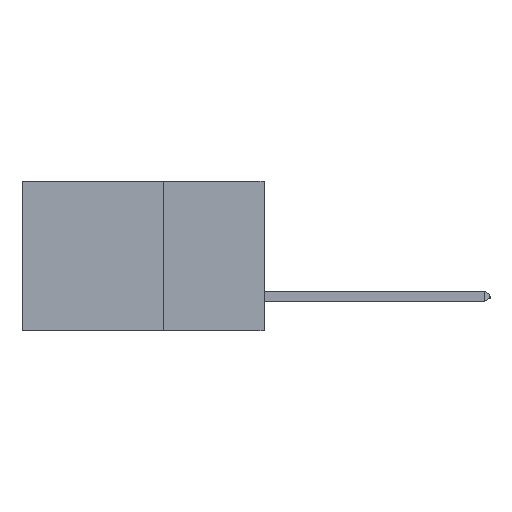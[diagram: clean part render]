
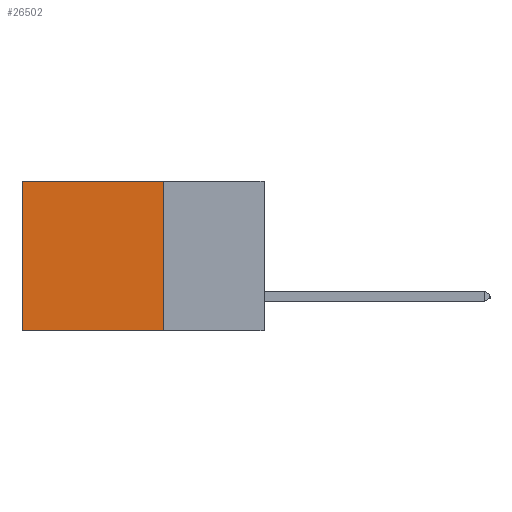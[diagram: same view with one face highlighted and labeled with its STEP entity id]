
A CAD part, left-side view. The second image highlights one B-rep face of the part: STEP entity #26502.
In plain terms, the highlighted planar face has unit normal (-1, 0, 0).
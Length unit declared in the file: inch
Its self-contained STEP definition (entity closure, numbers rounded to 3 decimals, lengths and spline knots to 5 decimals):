
#338 = CARTESIAN_POINT ( 'NONE',  ( 0.298, 0.25, -0.37 ) ) ;
#1048 = CARTESIAN_POINT ( 'NONE',  ( 0.298, 0.6, -0.37 ) ) ;
#1110 = CARTESIAN_POINT ( 'NONE',  ( 0.298, 0.25, 0. ) ) ;
#2152 = VERTEX_POINT ( 'NONE', #6720 ) ;
#2531 = DIRECTION ( 'NONE',  ( 0., 1., 0. ) ) ;
#2598 = VERTEX_POINT ( 'NONE', #15153 ) ;
#2757 = LINE ( 'NONE', #11496, #18764 ) ;
#3214 = PLANE ( 'NONE',  #15207 ) ;
#3659 = VECTOR ( 'NONE', #9325, 39.37008 ) ;
#4326 = LINE ( 'NONE', #7276, #3659 ) ;
#5459 = DIRECTION ( 'NONE',  ( 0., 0., -1. ) ) ;
#6161 = LINE ( 'NONE', #338, #26687 ) ;
#6407 = VERTEX_POINT ( 'NONE', #1048 ) ;
#6720 = CARTESIAN_POINT ( 'NONE',  ( 0.298, 0.25, 0. ) ) ;
#7276 = CARTESIAN_POINT ( 'NONE',  ( 0.298, 0.25, 0. ) ) ;
#7575 = EDGE_CURVE ( 'NONE', #2152, #7743, #4326, .T. ) ;
#7743 = VERTEX_POINT ( 'NONE', #18466 ) ;
#7853 = FACE_OUTER_BOUND ( 'NONE', #8866, .T. ) ;
#8143 = EDGE_CURVE ( 'NONE', #2152, #2598, #11509, .T. ) ;
#8866 = EDGE_LOOP ( 'NONE', ( #13284, #24932, #13434, #15311 ) ) ;
#9325 = DIRECTION ( 'NONE',  ( 0., 0., -1. ) ) ;
#11474 = DIRECTION ( 'NONE',  ( 0., 1., 0. ) ) ;
#11496 = CARTESIAN_POINT ( 'NONE',  ( 0.298, 0.6, 0. ) ) ;
#11509 = LINE ( 'NONE', #21656, #17054 ) ;
#13284 = ORIENTED_EDGE ( 'NONE', *, *, #13681, .T. ) ;
#13434 = ORIENTED_EDGE ( 'NONE', *, *, #7575, .F. ) ;
#13681 = EDGE_CURVE ( 'NONE', #2598, #6407, #2757, .T. ) ;
#15153 = CARTESIAN_POINT ( 'NONE',  ( 0.298, 0.6, 0. ) ) ;
#15207 = AXIS2_PLACEMENT_3D ( 'NONE', #1110, #17918, #5459 ) ;
#15311 = ORIENTED_EDGE ( 'NONE', *, *, #8143, .T. ) ;
#17054 = VECTOR ( 'NONE', #11474, 39.37008 ) ;
#17745 = DIRECTION ( 'NONE',  ( 0., 0., -1. ) ) ;
#17918 = DIRECTION ( 'NONE',  ( 1., 0., 0. ) ) ;
#18466 = CARTESIAN_POINT ( 'NONE',  ( 0.298, 0.25, -0.37 ) ) ;
#18764 = VECTOR ( 'NONE', #17745, 39.37008 ) ;
#21656 = CARTESIAN_POINT ( 'NONE',  ( 0.298, 0.25, 0. ) ) ;
#24932 = ORIENTED_EDGE ( 'NONE', *, *, #26798, .F. ) ;
#26502 = ADVANCED_FACE ( 'NONE', ( #7853 ), #3214, .F. ) ;
#26687 = VECTOR ( 'NONE', #2531, 39.37008 ) ;
#26798 = EDGE_CURVE ( 'NONE', #7743, #6407, #6161, .T. ) ;
